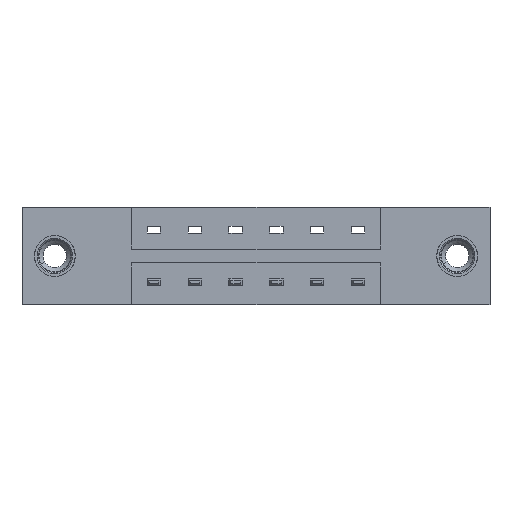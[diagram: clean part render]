
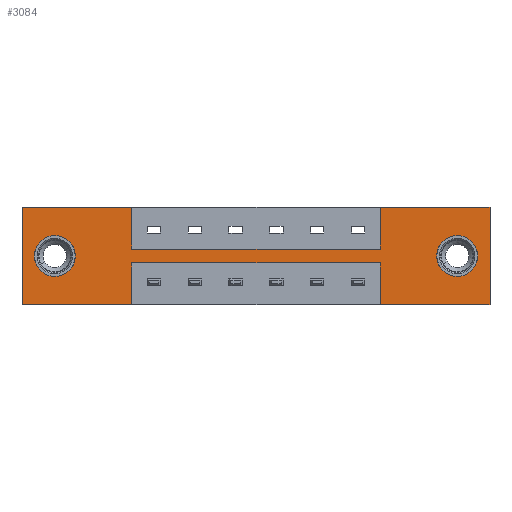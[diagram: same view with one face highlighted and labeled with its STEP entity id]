
A CAD part, front view. The second image highlights one B-rep face of the part: STEP entity #3084.
In plain terms, the highlighted planar face has unit normal (0, -1, 0).
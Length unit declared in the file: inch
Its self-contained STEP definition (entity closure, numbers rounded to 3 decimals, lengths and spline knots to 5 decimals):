
#70 = PLANE ( 'NONE',  #1924 ) ;
#153 = CARTESIAN_POINT ( 'NONE',  ( 0., 0., 0. ) ) ;
#178 = VECTOR ( 'NONE', #6300, 39.37008 ) ;
#183 = DIRECTION ( 'NONE',  ( 0., 0., 1. ) ) ;
#271 = CARTESIAN_POINT ( 'NONE',  ( 0.4175, 0., -0.1585 ) ) ;
#399 = CARTESIAN_POINT ( 'NONE',  ( 1.784, 0., -0.37 ) ) ;
#450 = AXIS2_PLACEMENT_3D ( 'NONE', #4991, #5583, #5617 ) ;
#603 = ORIENTED_EDGE ( 'NONE', *, *, #5419, .T. ) ;
#708 = EDGE_CURVE ( 'NONE', #8597, #2543, #9004, .T. ) ;
#709 = DIRECTION ( 'NONE',  ( 0., 0., -1. ) ) ;
#729 = VERTEX_POINT ( 'NONE', #5500 ) ;
#742 = VECTOR ( 'NONE', #4116, 39.37008 ) ;
#840 = ORIENTED_EDGE ( 'NONE', *, *, #3368, .F. ) ;
#1028 = VERTEX_POINT ( 'NONE', #8049 ) ;
#1066 = VERTEX_POINT ( 'NONE', #1116 ) ;
#1100 = EDGE_CURVE ( 'NONE', #9285, #5886, #5979, .T. ) ;
#1116 = CARTESIAN_POINT ( 'NONE',  ( 1.784, 0., 0. ) ) ;
#1153 = VECTOR ( 'NONE', #1417, 39.37008 ) ;
#1225 = EDGE_CURVE ( 'NONE', #1028, #8341, #3416, .T. ) ;
#1283 = LINE ( 'NONE', #1343, #3081 ) ;
#1315 = CARTESIAN_POINT ( 'NONE',  ( 1.659, 0., -0.263 ) ) ;
#1343 = CARTESIAN_POINT ( 'NONE',  ( 1.784, 0., 0. ) ) ;
#1417 = DIRECTION ( 'NONE',  ( 0., 0., -1. ) ) ;
#1420 = ORIENTED_EDGE ( 'NONE', *, *, #8911, .T. ) ;
#1548 = LINE ( 'NONE', #6688, #5209 ) ;
#1588 = CARTESIAN_POINT ( 'NONE',  ( 0.125, 0., -0.263 ) ) ;
#1603 = CARTESIAN_POINT ( 'NONE',  ( 1.3665, 0., -0.37 ) ) ;
#1681 = CARTESIAN_POINT ( 'NONE',  ( 1.3665, 0., -0.1585 ) ) ;
#1728 = LINE ( 'NONE', #7113, #3490 ) ;
#1841 = CIRCLE ( 'NONE', #5917, 0.078 ) ;
#1906 = CARTESIAN_POINT ( 'NONE',  ( 0., 0., -0.37 ) ) ;
#1924 = AXIS2_PLACEMENT_3D ( 'NONE', #9309, #9271, #9260 ) ;
#2098 = CARTESIAN_POINT ( 'NONE',  ( 0.125, 0., -0.185 ) ) ;
#2117 = DIRECTION ( 'NONE',  ( 0., 0., 1. ) ) ;
#2130 = DIRECTION ( 'NONE',  ( 0., 0., -1. ) ) ;
#2133 = VECTOR ( 'NONE', #709, 39.37008 ) ;
#2179 = ORIENTED_EDGE ( 'NONE', *, *, #1225, .T. ) ;
#2195 = VECTOR ( 'NONE', #2535, 39.37008 ) ;
#2299 = ORIENTED_EDGE ( 'NONE', *, *, #1100, .F. ) ;
#2416 = VERTEX_POINT ( 'NONE', #5154 ) ;
#2425 = LINE ( 'NONE', #6131, #2195 ) ;
#2464 = EDGE_CURVE ( 'NONE', #5886, #6939, #8045, .T. ) ;
#2477 = CARTESIAN_POINT ( 'NONE',  ( 0.4175, 0., -0.1585 ) ) ;
#2535 = DIRECTION ( 'NONE',  ( -1., 0., 0. ) ) ;
#2543 = VERTEX_POINT ( 'NONE', #3511 ) ;
#2824 = EDGE_CURVE ( 'NONE', #7142, #729, #9291, .T. ) ;
#2848 = DIRECTION ( 'NONE',  ( 0., 0., 1. ) ) ;
#3081 = VECTOR ( 'NONE', #2130, 39.37008 ) ;
#3084 = ADVANCED_FACE ( 'NONE', ( #9192, #7171, #8983 ), #70, .T. ) ;
#3098 = CARTESIAN_POINT ( 'NONE',  ( 1.659, 0., -0.185 ) ) ;
#3216 = EDGE_LOOP ( 'NONE', ( #4412, #840, #7476, #7288, #6250, #6305, #2299, #3960, #6883, #4235, #5060, #3461 ) ) ;
#3341 = EDGE_CURVE ( 'NONE', #2416, #8597, #8676, .T. ) ;
#3368 = EDGE_CURVE ( 'NONE', #3714, #4107, #8460, .T. ) ;
#3416 = CIRCLE ( 'NONE', #450, 0.078 ) ;
#3461 = ORIENTED_EDGE ( 'NONE', *, *, #3341, .F. ) ;
#3490 = VECTOR ( 'NONE', #2117, 39.37008 ) ;
#3511 = CARTESIAN_POINT ( 'NONE',  ( 0.4175, 0., -0.37 ) ) ;
#3714 = VERTEX_POINT ( 'NONE', #399 ) ;
#3735 = VECTOR ( 'NONE', #183, 39.37008 ) ;
#3785 = DIRECTION ( 'NONE',  ( 0., 1., 0. ) ) ;
#3815 = DIRECTION ( 'NONE',  ( 0., 0., -1. ) ) ;
#3846 = ORIENTED_EDGE ( 'NONE', *, *, #6817, .T. ) ;
#3960 = ORIENTED_EDGE ( 'NONE', *, *, #7997, .F. ) ;
#4107 = VERTEX_POINT ( 'NONE', #1603 ) ;
#4116 = DIRECTION ( 'NONE',  ( -1., 0., 0. ) ) ;
#4199 = LINE ( 'NONE', #5573, #178 ) ;
#4235 = ORIENTED_EDGE ( 'NONE', *, *, #9053, .F. ) ;
#4296 = DIRECTION ( 'NONE',  ( 0., 0., 1. ) ) ;
#4412 = ORIENTED_EDGE ( 'NONE', *, *, #8124, .F. ) ;
#4518 = DIRECTION ( 'NONE',  ( 1., 0., 0. ) ) ;
#4558 = DIRECTION ( 'NONE',  ( -1., 0., 0. ) ) ;
#4599 = CARTESIAN_POINT ( 'NONE',  ( 0., 0., -0.37 ) ) ;
#4606 = CARTESIAN_POINT ( 'NONE',  ( 0.4175, 0., -0.1585 ) ) ;
#4738 = CARTESIAN_POINT ( 'NONE',  ( 0.4175, 0., -0.2115 ) ) ;
#4785 = CIRCLE ( 'NONE', #5469, 0.078 ) ;
#4942 = VECTOR ( 'NONE', #4558, 39.37008 ) ;
#4991 = CARTESIAN_POINT ( 'NONE',  ( 0.125, 0., -0.185 ) ) ;
#5041 = CARTESIAN_POINT ( 'NONE',  ( 0.4175, 0., -0.2115 ) ) ;
#5060 = ORIENTED_EDGE ( 'NONE', *, *, #708, .F. ) ;
#5154 = CARTESIAN_POINT ( 'NONE',  ( 1.3665, 0., -0.2115 ) ) ;
#5209 = VECTOR ( 'NONE', #7368, 39.37008 ) ;
#5419 = EDGE_CURVE ( 'NONE', #8341, #1028, #4785, .T. ) ;
#5427 = VERTEX_POINT ( 'NONE', #1315 ) ;
#5469 = AXIS2_PLACEMENT_3D ( 'NONE', #2098, #7127, #2848 ) ;
#5500 = CARTESIAN_POINT ( 'NONE',  ( 0., 0., 0. ) ) ;
#5573 = CARTESIAN_POINT ( 'NONE',  ( 0., 0., 0. ) ) ;
#5583 = DIRECTION ( 'NONE',  ( 0., 1., 0. ) ) ;
#5617 = DIRECTION ( 'NONE',  ( 0., 0., 1. ) ) ;
#5816 = EDGE_LOOP ( 'NONE', ( #1420, #3846 ) ) ;
#5886 = VERTEX_POINT ( 'NONE', #271 ) ;
#5917 = AXIS2_PLACEMENT_3D ( 'NONE', #3098, #8040, #3815 ) ;
#5979 = LINE ( 'NONE', #2477, #2133 ) ;
#6131 = CARTESIAN_POINT ( 'NONE',  ( 0., 0., -0.37 ) ) ;
#6200 = VECTOR ( 'NONE', #4518, 39.37008 ) ;
#6250 = ORIENTED_EDGE ( 'NONE', *, *, #8708, .F. ) ;
#6300 = DIRECTION ( 'NONE',  ( 1., 0., 0. ) ) ;
#6305 = ORIENTED_EDGE ( 'NONE', *, *, #2464, .F. ) ;
#6688 = CARTESIAN_POINT ( 'NONE',  ( 0., 0., 0. ) ) ;
#6766 = CARTESIAN_POINT ( 'NONE',  ( 1.659, 0., -0.107 ) ) ;
#6817 = EDGE_CURVE ( 'NONE', #5427, #8437, #9224, .T. ) ;
#6883 = ORIENTED_EDGE ( 'NONE', *, *, #2824, .F. ) ;
#6939 = VERTEX_POINT ( 'NONE', #1681 ) ;
#7087 = LINE ( 'NONE', #9173, #8711 ) ;
#7113 = CARTESIAN_POINT ( 'NONE',  ( 1.3665, 0., -0.1585 ) ) ;
#7127 = DIRECTION ( 'NONE',  ( 0., 1., 0. ) ) ;
#7142 = VERTEX_POINT ( 'NONE', #1906 ) ;
#7171 = FACE_BOUND ( 'NONE', #7425, .T. ) ;
#7193 = CARTESIAN_POINT ( 'NONE',  ( 0.4175, 0., 0. ) ) ;
#7288 = ORIENTED_EDGE ( 'NONE', *, *, #7711, .F. ) ;
#7368 = DIRECTION ( 'NONE',  ( 1., 0., 0. ) ) ;
#7396 = VERTEX_POINT ( 'NONE', #7965 ) ;
#7425 = EDGE_LOOP ( 'NONE', ( #2179, #603 ) ) ;
#7476 = ORIENTED_EDGE ( 'NONE', *, *, #8126, .F. ) ;
#7595 = AXIS2_PLACEMENT_3D ( 'NONE', #8002, #3785, #8706 ) ;
#7711 = EDGE_CURVE ( 'NONE', #7396, #1066, #1548, .T. ) ;
#7965 = CARTESIAN_POINT ( 'NONE',  ( 1.3665, 0., 0. ) ) ;
#7997 = EDGE_CURVE ( 'NONE', #729, #9285, #4199, .T. ) ;
#8002 = CARTESIAN_POINT ( 'NONE',  ( 1.659, 0., -0.185 ) ) ;
#8040 = DIRECTION ( 'NONE',  ( 0., 1., 0. ) ) ;
#8045 = LINE ( 'NONE', #4606, #6200 ) ;
#8049 = CARTESIAN_POINT ( 'NONE',  ( 0.125, 0., -0.107 ) ) ;
#8124 = EDGE_CURVE ( 'NONE', #4107, #2416, #7087, .T. ) ;
#8126 = EDGE_CURVE ( 'NONE', #1066, #3714, #1283, .T. ) ;
#8341 = VERTEX_POINT ( 'NONE', #1588 ) ;
#8350 = CARTESIAN_POINT ( 'NONE',  ( 0.4175, 0., -0.2115 ) ) ;
#8437 = VERTEX_POINT ( 'NONE', #6766 ) ;
#8460 = LINE ( 'NONE', #4599, #742 ) ;
#8597 = VERTEX_POINT ( 'NONE', #8350 ) ;
#8676 = LINE ( 'NONE', #5041, #4942 ) ;
#8706 = DIRECTION ( 'NONE',  ( 0., 0., -1. ) ) ;
#8708 = EDGE_CURVE ( 'NONE', #6939, #7396, #1728, .T. ) ;
#8711 = VECTOR ( 'NONE', #4296, 39.37008 ) ;
#8911 = EDGE_CURVE ( 'NONE', #8437, #5427, #1841, .T. ) ;
#8983 = FACE_OUTER_BOUND ( 'NONE', #3216, .T. ) ;
#9004 = LINE ( 'NONE', #4738, #1153 ) ;
#9053 = EDGE_CURVE ( 'NONE', #2543, #7142, #2425, .T. ) ;
#9173 = CARTESIAN_POINT ( 'NONE',  ( 1.3665, 0., -0.2115 ) ) ;
#9192 = FACE_BOUND ( 'NONE', #5816, .T. ) ;
#9224 = CIRCLE ( 'NONE', #7595, 0.078 ) ;
#9260 = DIRECTION ( 'NONE',  ( 0., 0., -1. ) ) ;
#9271 = DIRECTION ( 'NONE',  ( 0., -1., 0. ) ) ;
#9285 = VERTEX_POINT ( 'NONE', #7193 ) ;
#9291 = LINE ( 'NONE', #153, #3735 ) ;
#9309 = CARTESIAN_POINT ( 'NONE',  ( 0., 0., -0.37 ) ) ;
